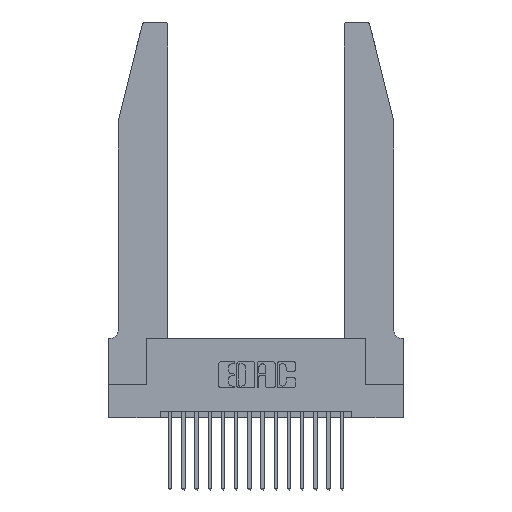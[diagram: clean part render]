
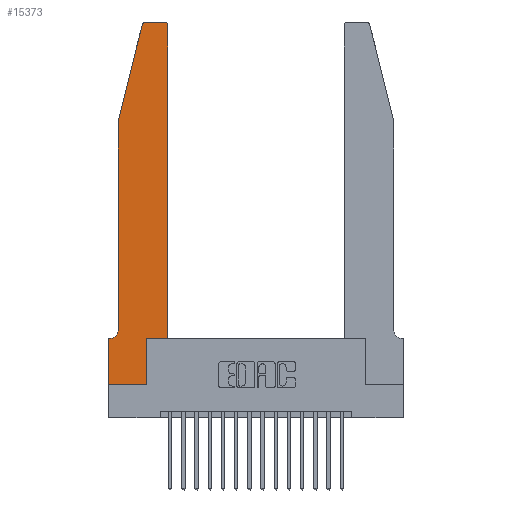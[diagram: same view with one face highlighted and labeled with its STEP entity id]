
A CAD part, top view. The second image highlights one B-rep face of the part: STEP entity #15373.
In plain terms, the highlighted planar face has unit normal (0, 0, 1).
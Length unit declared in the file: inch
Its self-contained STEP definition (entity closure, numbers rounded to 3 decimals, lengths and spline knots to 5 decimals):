
#369 = EDGE_CURVE ( 'NONE', #5362, #14354, #13733, .T. ) ;
#800 = EDGE_CURVE ( 'NONE', #10596, #8719, #4015, .T. ) ;
#919 = LINE ( 'NONE', #14676, #12688 ) ;
#925 = EDGE_CURVE ( 'NONE', #13363, #10596, #2064, .T. ) ;
#987 = CARTESIAN_POINT ( 'NONE',  ( 0.0755, 2., 0.37 ) ) ;
#1285 = CARTESIAN_POINT ( 'NONE',  ( 0.0755, 2., 0.37 ) ) ;
#1416 = CARTESIAN_POINT ( 'NONE',  ( 0.2865, 0.35, 0.37 ) ) ;
#1451 = EDGE_CURVE ( 'NONE', #8719, #5362, #6170, .T. ) ;
#1501 = ORIENTED_EDGE ( 'NONE', *, *, #11888, .T. ) ;
#2064 = CIRCLE ( 'NONE', #14331, 0.03 ) ;
#2152 = VERTEX_POINT ( 'NONE', #17757 ) ;
#2540 = VECTOR ( 'NONE', #3390, 39.37008 ) ;
#2934 = VERTEX_POINT ( 'NONE', #12129 ) ;
#3024 = DIRECTION ( 'NONE',  ( 0., 1., 0. ) ) ;
#3300 = AXIS2_PLACEMENT_3D ( 'NONE', #8416, #18668, #9936 ) ;
#3390 = DIRECTION ( 'NONE',  ( 0., -1., 0. ) ) ;
#3415 = CARTESIAN_POINT ( 'NONE',  ( 0.0755, 2., 0.37 ) ) ;
#3719 = VECTOR ( 'NONE', #17886, 39.37008 ) ;
#3817 = CARTESIAN_POINT ( 'NONE',  ( 0.284, 2.75, 0.37 ) ) ;
#3962 = VERTEX_POINT ( 'NONE', #17261 ) ;
#4015 = LINE ( 'NONE', #987, #18885 ) ;
#4148 = VERTEX_POINT ( 'NONE', #14759 ) ;
#4154 = EDGE_CURVE ( 'NONE', #2934, #13363, #6140, .T. ) ;
#4165 = DIRECTION ( 'NONE',  ( 0., 1., 0. ) ) ;
#4209 = LINE ( 'NONE', #5997, #3719 ) ;
#4223 = ORIENTED_EDGE ( 'NONE', *, *, #6273, .T. ) ;
#4226 = EDGE_CURVE ( 'NONE', #10898, #3962, #4209, .T. ) ;
#4547 = DIRECTION ( 'NONE',  ( 0., -1., 0. ) ) ;
#5362 = VERTEX_POINT ( 'NONE', #18428 ) ;
#5997 = CARTESIAN_POINT ( 'NONE',  ( 0.4505, 0.35, 0.37 ) ) ;
#6140 = LINE ( 'NONE', #8875, #16643 ) ;
#6170 = LINE ( 'NONE', #3415, #2540 ) ;
#6246 = ORIENTED_EDGE ( 'NONE', *, *, #12539, .T. ) ;
#6273 = EDGE_CURVE ( 'NONE', #3962, #9966, #919, .T. ) ;
#6355 = CARTESIAN_POINT ( 'NONE',  ( 0.4505, 2.72, 0.37 ) ) ;
#6665 = CARTESIAN_POINT ( 'NONE',  ( 0.0055, 0.35, 0.37 ) ) ;
#6695 = AXIS2_PLACEMENT_3D ( 'NONE', #7893, #7870, #8249 ) ;
#6765 = CARTESIAN_POINT ( 'NONE',  ( 0.0755, 0.35, 0.37 ) ) ;
#6825 = EDGE_CURVE ( 'NONE', #14354, #10846, #12666, .T. ) ;
#7092 = DIRECTION ( 'NONE',  ( -0.239, -0.971, 0. ) ) ;
#7132 = DIRECTION ( 'NONE',  ( 0., 0., 1. ) ) ;
#7368 = CARTESIAN_POINT ( 'NONE',  ( 0.284, 2.72, 0.37 ) ) ;
#7551 = CARTESIAN_POINT ( 'NONE',  ( 0., 0.35, 0.37 ) ) ;
#7600 = ORIENTED_EDGE ( 'NONE', *, *, #15596, .T. ) ;
#7870 = DIRECTION ( 'NONE',  ( 0., 0., -1. ) ) ;
#7893 = CARTESIAN_POINT ( 'NONE',  ( 0.0055, 0.42, 0.37 ) ) ;
#7963 = CARTESIAN_POINT ( 'NONE',  ( 0.2865, 0.35, 0.37 ) ) ;
#8249 = DIRECTION ( 'NONE',  ( -1., 0., 0. ) ) ;
#8416 = CARTESIAN_POINT ( 'NONE',  ( 0.4205, 2.72, 0.37 ) ) ;
#8578 = EDGE_LOOP ( 'NONE', ( #14114, #11009, #19352, #18432, #14887, #11226, #6246, #8691, #1501, #18566, #4223, #7600 ) ) ;
#8691 = ORIENTED_EDGE ( 'NONE', *, *, #10810, .T. ) ;
#8719 = VERTEX_POINT ( 'NONE', #1285 ) ;
#8875 = CARTESIAN_POINT ( 'NONE',  ( 0.2605, 2.75, 0.37 ) ) ;
#9105 = DIRECTION ( 'NONE',  ( 1., 0., 0. ) ) ;
#9305 = DIRECTION ( 'NONE',  ( 1., 0., 0. ) ) ;
#9541 = DIRECTION ( 'NONE',  ( 1., 0., 0. ) ) ;
#9936 = DIRECTION ( 'NONE',  ( 1., 0., 0. ) ) ;
#9966 = VERTEX_POINT ( 'NONE', #6355 ) ;
#10596 = VERTEX_POINT ( 'NONE', #14666 ) ;
#10810 = EDGE_CURVE ( 'NONE', #4148, #2152, #13870, .T. ) ;
#10828 = LINE ( 'NONE', #12100, #17667 ) ;
#10840 = FACE_OUTER_BOUND ( 'NONE', #8578, .T. ) ;
#10846 = VERTEX_POINT ( 'NONE', #13779 ) ;
#10898 = VERTEX_POINT ( 'NONE', #7963 ) ;
#11009 = ORIENTED_EDGE ( 'NONE', *, *, #925, .T. ) ;
#11226 = ORIENTED_EDGE ( 'NONE', *, *, #6825, .T. ) ;
#11750 = DIRECTION ( 'NONE',  ( -1., 0., 0. ) ) ;
#11888 = EDGE_CURVE ( 'NONE', #2152, #10898, #13609, .T. ) ;
#12100 = CARTESIAN_POINT ( 'NONE',  ( 0., 0., 0.37 ) ) ;
#12129 = CARTESIAN_POINT ( 'NONE',  ( 0.4205, 2.75, 0.37 ) ) ;
#12539 = EDGE_CURVE ( 'NONE', #10846, #4148, #10828, .T. ) ;
#12666 = LINE ( 'NONE', #6765, #15636 ) ;
#12688 = VECTOR ( 'NONE', #4165, 39.37008 ) ;
#13133 = VECTOR ( 'NONE', #3024, 39.37008 ) ;
#13363 = VERTEX_POINT ( 'NONE', #3817 ) ;
#13609 = LINE ( 'NONE', #1416, #13133 ) ;
#13733 = CIRCLE ( 'NONE', #6695, 0.07 ) ;
#13779 = CARTESIAN_POINT ( 'NONE',  ( 0., 0.35, 0.37 ) ) ;
#13810 = AXIS2_PLACEMENT_3D ( 'NONE', #7551, #17902, #9105 ) ;
#13870 = LINE ( 'NONE', #16667, #16848 ) ;
#14021 = CIRCLE ( 'NONE', #3300, 0.03 ) ;
#14114 = ORIENTED_EDGE ( 'NONE', *, *, #4154, .T. ) ;
#14331 = AXIS2_PLACEMENT_3D ( 'NONE', #7368, #7132, #9541 ) ;
#14339 = DIRECTION ( 'NONE',  ( -1., 0., 0. ) ) ;
#14354 = VERTEX_POINT ( 'NONE', #6665 ) ;
#14666 = CARTESIAN_POINT ( 'NONE',  ( 0.25487, 2.72718, 0.37 ) ) ;
#14676 = CARTESIAN_POINT ( 'NONE',  ( 0.4505, 0.35, 0.37 ) ) ;
#14759 = CARTESIAN_POINT ( 'NONE',  ( 0., 0., 0.37 ) ) ;
#14887 = ORIENTED_EDGE ( 'NONE', *, *, #369, .T. ) ;
#15373 = ADVANCED_FACE ( 'NONE', ( #10840 ), #16463, .T. ) ;
#15596 = EDGE_CURVE ( 'NONE', #9966, #2934, #14021, .T. ) ;
#15636 = VECTOR ( 'NONE', #14339, 39.37008 ) ;
#16463 = PLANE ( 'NONE',  #13810 ) ;
#16643 = VECTOR ( 'NONE', #11750, 39.37008 ) ;
#16667 = CARTESIAN_POINT ( 'NONE',  ( 0., 0., 0.37 ) ) ;
#16848 = VECTOR ( 'NONE', #9305, 39.37008 ) ;
#17261 = CARTESIAN_POINT ( 'NONE',  ( 0.4505, 0.35, 0.37 ) ) ;
#17667 = VECTOR ( 'NONE', #4547, 39.37008 ) ;
#17757 = CARTESIAN_POINT ( 'NONE',  ( 0.2865, 0., 0.37 ) ) ;
#17886 = DIRECTION ( 'NONE',  ( 1., 0., 0. ) ) ;
#17902 = DIRECTION ( 'NONE',  ( 0., 0., 1. ) ) ;
#18428 = CARTESIAN_POINT ( 'NONE',  ( 0.0755, 0.42, 0.37 ) ) ;
#18432 = ORIENTED_EDGE ( 'NONE', *, *, #1451, .T. ) ;
#18566 = ORIENTED_EDGE ( 'NONE', *, *, #4226, .T. ) ;
#18668 = DIRECTION ( 'NONE',  ( 0., 0., 1. ) ) ;
#18885 = VECTOR ( 'NONE', #7092, 39.37008 ) ;
#19352 = ORIENTED_EDGE ( 'NONE', *, *, #800, .T. ) ;
